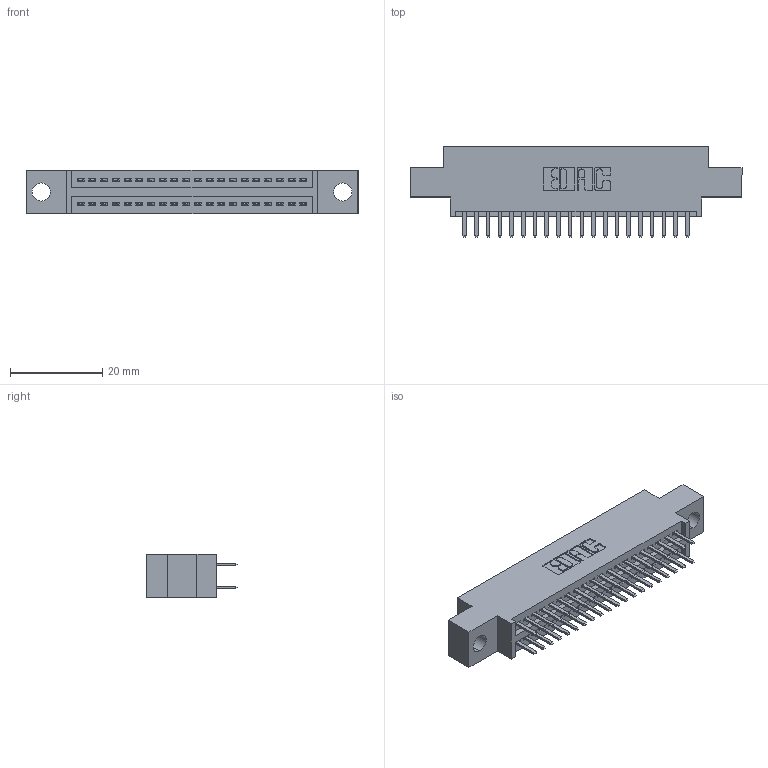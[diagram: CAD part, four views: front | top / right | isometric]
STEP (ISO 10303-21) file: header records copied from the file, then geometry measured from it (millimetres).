
FILE_DESCRIPTION (( 'STEP AP203' ), '1' );
FILE_NAME ('345-040-520-804.STEP', '2021-05-20T01:03:18', ( '' ), ( '' ), 'SwSTEP 2.0', 'SolidWorks 2020', '' );
FILE_SCHEMA (( 'CONFIG_CONTROL_DESIGN' ));
Length unit declared in the file: inch
Products named in the file (3): 345 Part_0.170 Offset - 0.156 Dia-TI; 345-040-520-804; 345-292-001_345-293-120
Assembly tree (41 placements, depth 2):
  345-040-520-804
    345 Part_0.170 Offset - 0.156 Dia-TI
    345-292-001_345-293-120  x40
Bounding box: 72.01 x 19.68 x 9.4 mm (x, y, z)
Volume: 6553.9 mm3; surface area: 9219.3 mm2
Topology: 41 solids, 41 shells, 2304 faces, 6669 edges, 4338 vertices
Faces by surface type: plane 1498, cylinder 806
Entity records: 19319 total; most frequent: CARTESIAN_POINT 3278, ORIENTED_EDGE 3198, DIRECTION 2903, EDGE_CURVE 1599, LINE 1383, VECTOR 1383, VERTEX_POINT 1062, AXIS2_PLACEMENT_3D 760
